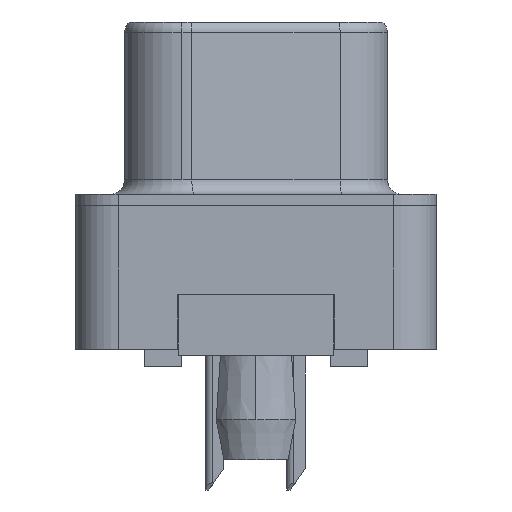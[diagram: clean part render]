
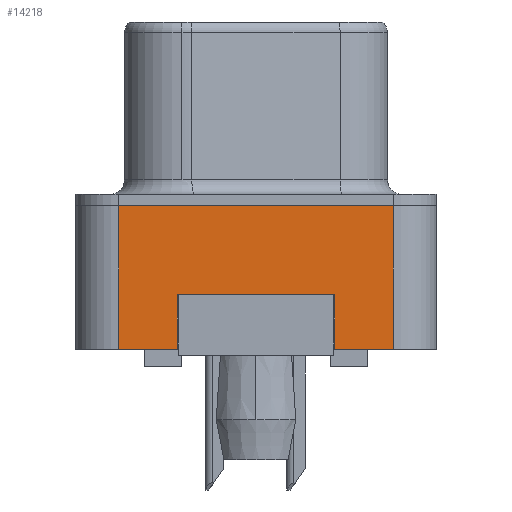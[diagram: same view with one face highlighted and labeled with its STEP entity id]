
A CAD part, left-side view. The second image highlights one B-rep face of the part: STEP entity #14218.
In plain terms, the highlighted planar face has unit normal (-1, 0, 0).
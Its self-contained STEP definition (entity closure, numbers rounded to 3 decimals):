
#181 = CARTESIAN_POINT ( 'NONE',  ( -2.935, -4.775, -5. ) ) ;
#905 = DIRECTION ( 'NONE',  ( 0., 1., 0. ) ) ;
#1280 = CARTESIAN_POINT ( 'NONE',  ( -2.935, 4.775, 0. ) ) ;
#1348 = ORIENTED_EDGE ( 'NONE', *, *, #8364, .T. ) ;
#1367 = CARTESIAN_POINT ( 'NONE',  ( -2.935, -4.775, -5. ) ) ;
#1384 = CARTESIAN_POINT ( 'NONE',  ( -2.935, 2.75, -3.1 ) ) ;
#1900 = VERTEX_POINT ( 'NONE', #3111 ) ;
#2123 = ORIENTED_EDGE ( 'NONE', *, *, #11148, .T. ) ;
#2171 = CARTESIAN_POINT ( 'NONE',  ( -2.935, -4.775, 0. ) ) ;
#2567 = ORIENTED_EDGE ( 'NONE', *, *, #8832, .T. ) ;
#2969 = DIRECTION ( 'NONE',  ( -1., 0., 0. ) ) ;
#2971 = VERTEX_POINT ( 'NONE', #7610 ) ;
#3111 = CARTESIAN_POINT ( 'NONE',  ( -2.935, -2.75, -3.1 ) ) ;
#3374 = CARTESIAN_POINT ( 'NONE',  ( -2.935, -2.75, -3.1 ) ) ;
#3418 = VERTEX_POINT ( 'NONE', #3540 ) ;
#3448 = EDGE_CURVE ( 'NONE', #3418, #12897, #6992, .T. ) ;
#3469 = VECTOR ( 'NONE', #11255, 1000. ) ;
#3526 = LINE ( 'NONE', #13706, #4051 ) ;
#3540 = CARTESIAN_POINT ( 'NONE',  ( -2.935, 2.75, -3.1 ) ) ;
#3584 = EDGE_LOOP ( 'NONE', ( #2123, #2567, #14365, #7418, #11000, #1348, #14456, #11254 ) ) ;
#3625 = VERTEX_POINT ( 'NONE', #11836 ) ;
#4051 = VECTOR ( 'NONE', #905, 1000. ) ;
#4135 = VECTOR ( 'NONE', #9072, 1000. ) ;
#4237 = LINE ( 'NONE', #9929, #3469 ) ;
#4287 = DIRECTION ( 'NONE',  ( 0., -1., 0. ) ) ;
#5492 = VECTOR ( 'NONE', #15873, 1000. ) ;
#5684 = CARTESIAN_POINT ( 'NONE',  ( -2.935, -4.775, -5. ) ) ;
#6142 = VECTOR ( 'NONE', #14172, 1000. ) ;
#6761 = AXIS2_PLACEMENT_3D ( 'NONE', #5684, #2969, #14457 ) ;
#6992 = LINE ( 'NONE', #1384, #14461 ) ;
#7180 = PLANE ( 'NONE',  #6761 ) ;
#7276 = LINE ( 'NONE', #9980, #5492 ) ;
#7418 = ORIENTED_EDGE ( 'NONE', *, *, #7940, .F. ) ;
#7610 = CARTESIAN_POINT ( 'NONE',  ( -2.935, 4.775, -5. ) ) ;
#7940 = EDGE_CURVE ( 'NONE', #9224, #9575, #7276, .T. ) ;
#7943 = VERTEX_POINT ( 'NONE', #181 ) ;
#8267 = EDGE_CURVE ( 'NONE', #1900, #3418, #3526, .T. ) ;
#8364 = EDGE_CURVE ( 'NONE', #2971, #12897, #11361, .T. ) ;
#8591 = CARTESIAN_POINT ( 'NONE',  ( -2.935, -4.775, -5. ) ) ;
#8832 = EDGE_CURVE ( 'NONE', #3625, #7943, #14204, .T. ) ;
#9072 = DIRECTION ( 'NONE',  ( 0., 0., -1. ) ) ;
#9224 = VERTEX_POINT ( 'NONE', #1280 ) ;
#9575 = VERTEX_POINT ( 'NONE', #2171 ) ;
#9929 = CARTESIAN_POINT ( 'NONE',  ( -2.935, 4.775, -5. ) ) ;
#9980 = CARTESIAN_POINT ( 'NONE',  ( -2.935, -4.775, 0. ) ) ;
#10388 = LINE ( 'NONE', #3374, #4135 ) ;
#11000 = ORIENTED_EDGE ( 'NONE', *, *, #18198, .F. ) ;
#11148 = EDGE_CURVE ( 'NONE', #1900, #3625, #10388, .T. ) ;
#11197 = DIRECTION ( 'NONE',  ( 0., 0., -1. ) ) ;
#11254 = ORIENTED_EDGE ( 'NONE', *, *, #8267, .F. ) ;
#11255 = DIRECTION ( 'NONE',  ( 0., 0., 1. ) ) ;
#11361 = LINE ( 'NONE', #1367, #6142 ) ;
#11589 = DIRECTION ( 'NONE',  ( 0., 0., 1. ) ) ;
#11831 = VECTOR ( 'NONE', #4287, 1000. ) ;
#11836 = CARTESIAN_POINT ( 'NONE',  ( -2.935, -2.75, -5. ) ) ;
#12305 = VECTOR ( 'NONE', #11589, 1000. ) ;
#12407 = CARTESIAN_POINT ( 'NONE',  ( -2.935, 2.75, -5. ) ) ;
#12804 = CARTESIAN_POINT ( 'NONE',  ( -2.935, -4.775, -5. ) ) ;
#12897 = VERTEX_POINT ( 'NONE', #12407 ) ;
#13706 = CARTESIAN_POINT ( 'NONE',  ( -2.935, 2.75, -3.1 ) ) ;
#14172 = DIRECTION ( 'NONE',  ( 0., -1., 0. ) ) ;
#14204 = LINE ( 'NONE', #8591, #11831 ) ;
#14218 = ADVANCED_FACE ( 'NONE', ( #14366 ), #7180, .T. ) ;
#14365 = ORIENTED_EDGE ( 'NONE', *, *, #16922, .T. ) ;
#14366 = FACE_OUTER_BOUND ( 'NONE', #3584, .T. ) ;
#14456 = ORIENTED_EDGE ( 'NONE', *, *, #3448, .F. ) ;
#14457 = DIRECTION ( 'NONE',  ( 0., 0., 1. ) ) ;
#14461 = VECTOR ( 'NONE', #11197, 1000. ) ;
#15873 = DIRECTION ( 'NONE',  ( 0., -1., 0. ) ) ;
#16922 = EDGE_CURVE ( 'NONE', #7943, #9575, #17299, .T. ) ;
#17299 = LINE ( 'NONE', #12804, #12305 ) ;
#18198 = EDGE_CURVE ( 'NONE', #2971, #9224, #4237, .T. ) ;
